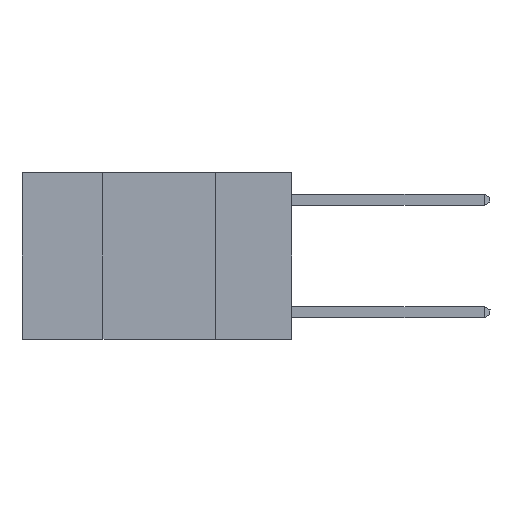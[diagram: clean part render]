
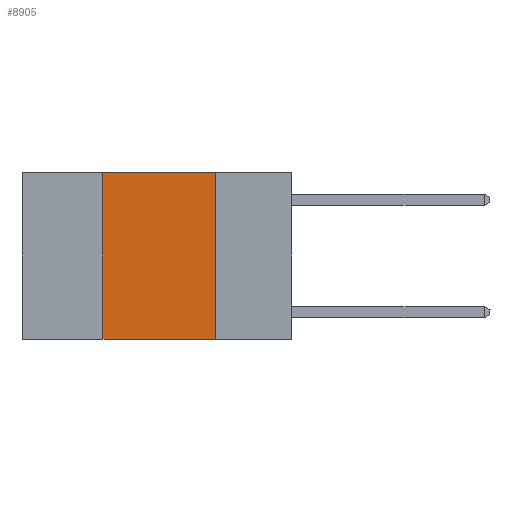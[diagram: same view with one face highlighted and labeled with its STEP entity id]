
A CAD part, left-side view. The second image highlights one B-rep face of the part: STEP entity #8905.
In plain terms, the highlighted planar face has unit normal (-1, 0, 0).
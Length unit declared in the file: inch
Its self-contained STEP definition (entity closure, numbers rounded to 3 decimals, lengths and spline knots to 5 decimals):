
#116 = VERTEX_POINT ( 'NONE', #1287 ) ;
#1008 = LINE ( 'NONE', #6436, #10281 ) ;
#1287 = CARTESIAN_POINT ( 'NONE',  ( 0., 0.17, 0. ) ) ;
#1310 = EDGE_CURVE ( 'NONE', #3172, #10337, #8738, .T. ) ;
#2202 = LINE ( 'NONE', #9370, #8692 ) ;
#2316 = ORIENTED_EDGE ( 'NONE', *, *, #8757, .F. ) ;
#2427 = CARTESIAN_POINT ( 'NONE',  ( 0., 0.17, -0.37 ) ) ;
#2904 = CARTESIAN_POINT ( 'NONE',  ( 0., 0.6, 0. ) ) ;
#2986 = AXIS2_PLACEMENT_3D ( 'NONE', #2904, #10401, #5480 ) ;
#3172 = VERTEX_POINT ( 'NONE', #8374 ) ;
#3425 = CARTESIAN_POINT ( 'NONE',  ( 0., 0.42, 0. ) ) ;
#3559 = DIRECTION ( 'NONE',  ( 0., 0., -1. ) ) ;
#3598 = CARTESIAN_POINT ( 'NONE',  ( 0., 0.42, 0. ) ) ;
#3659 = EDGE_CURVE ( 'NONE', #9268, #116, #1008, .T. ) ;
#3843 = ORIENTED_EDGE ( 'NONE', *, *, #7914, .F. ) ;
#4343 = DIRECTION ( 'NONE',  ( 0., -1., 0. ) ) ;
#4344 = CARTESIAN_POINT ( 'NONE',  ( 0., 0.6, -0.37 ) ) ;
#4497 = LINE ( 'NONE', #3598, #6707 ) ;
#4640 = PLANE ( 'NONE',  #2986 ) ;
#4709 = EDGE_LOOP ( 'NONE', ( #3843, #8797, #2316, #6820 ) ) ;
#5141 = FACE_OUTER_BOUND ( 'NONE', #4709, .T. ) ;
#5480 = DIRECTION ( 'NONE',  ( 0., 0., -1. ) ) ;
#6260 = VECTOR ( 'NONE', #4343, 39.37008 ) ;
#6436 = CARTESIAN_POINT ( 'NONE',  ( 0., 0.6, 0. ) ) ;
#6707 = VECTOR ( 'NONE', #7730, 39.37008 ) ;
#6820 = ORIENTED_EDGE ( 'NONE', *, *, #1310, .T. ) ;
#7730 = DIRECTION ( 'NONE',  ( 0., 0., 1. ) ) ;
#7914 = EDGE_CURVE ( 'NONE', #116, #10337, #2202, .T. ) ;
#8374 = CARTESIAN_POINT ( 'NONE',  ( 0., 0.42, -0.37 ) ) ;
#8692 = VECTOR ( 'NONE', #3559, 39.37008 ) ;
#8738 = LINE ( 'NONE', #4344, #6260 ) ;
#8757 = EDGE_CURVE ( 'NONE', #3172, #9268, #4497, .T. ) ;
#8797 = ORIENTED_EDGE ( 'NONE', *, *, #3659, .F. ) ;
#8905 = ADVANCED_FACE ( 'NONE', ( #5141 ), #4640, .F. ) ;
#9268 = VERTEX_POINT ( 'NONE', #3425 ) ;
#9370 = CARTESIAN_POINT ( 'NONE',  ( 0., 0.17, 0. ) ) ;
#10281 = VECTOR ( 'NONE', #10528, 39.37008 ) ;
#10337 = VERTEX_POINT ( 'NONE', #2427 ) ;
#10401 = DIRECTION ( 'NONE',  ( 1., 0., 0. ) ) ;
#10528 = DIRECTION ( 'NONE',  ( 0., -1., 0. ) ) ;
